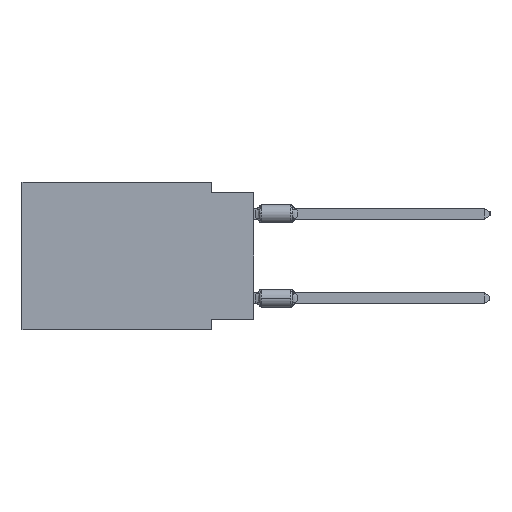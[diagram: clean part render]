
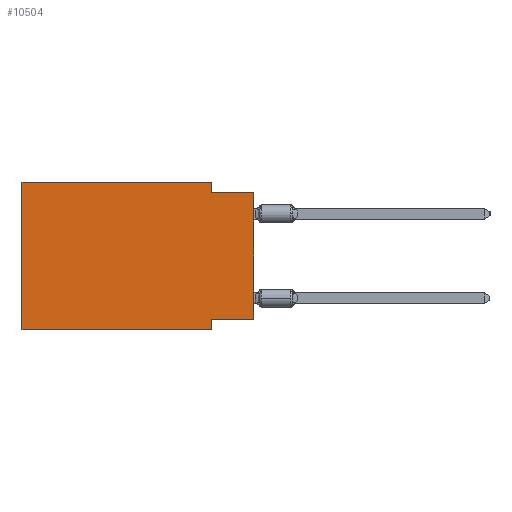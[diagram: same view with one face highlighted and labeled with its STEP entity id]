
A CAD part, left-side view. The second image highlights one B-rep face of the part: STEP entity #10504.
In plain terms, the highlighted planar face has unit normal (-1, 0, 0).
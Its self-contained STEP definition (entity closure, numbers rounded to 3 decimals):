
#73 = VERTEX_POINT ( 'NONE', #5801 ) ;
#1400 = CARTESIAN_POINT ( 'NONE',  ( 0., 13.97, -8.89 ) ) ;
#1407 = CARTESIAN_POINT ( 'NONE',  ( 0., 2.54, 0. ) ) ;
#2314 = EDGE_CURVE ( 'NONE', #11954, #22355, #8105, .T. ) ;
#2711 = ORIENTED_EDGE ( 'NONE', *, *, #22568, .F. ) ;
#4133 = VERTEX_POINT ( 'NONE', #24813 ) ;
#5801 = CARTESIAN_POINT ( 'NONE',  ( 0., 13.97, 0. ) ) ;
#6069 = CARTESIAN_POINT ( 'NONE',  ( 0., 13.97, 0. ) ) ;
#6462 = EDGE_CURVE ( 'NONE', #14252, #42891, #11161, .T. ) ;
#7200 = CARTESIAN_POINT ( 'NONE',  ( 0., 0., 0. ) ) ;
#8105 = LINE ( 'NONE', #1400, #47769 ) ;
#9784 = LINE ( 'NONE', #6069, #10250 ) ;
#9906 = FACE_OUTER_BOUND ( 'NONE', #31492, .T. ) ;
#10010 = EDGE_CURVE ( 'NONE', #11954, #73, #9784, .T. ) ;
#10250 = VECTOR ( 'NONE', #39544, 1000. ) ;
#10504 = ADVANCED_FACE ( 'NONE', ( #9906 ), #32223, .F. ) ;
#11161 = LINE ( 'NONE', #7200, #14114 ) ;
#11415 = ORIENTED_EDGE ( 'NONE', *, *, #10010, .F. ) ;
#11954 = VERTEX_POINT ( 'NONE', #25848 ) ;
#13137 = DIRECTION ( 'NONE',  ( 1., 0., 0. ) ) ;
#13184 = ORIENTED_EDGE ( 'NONE', *, *, #28452, .F. ) ;
#13255 = EDGE_CURVE ( 'NONE', #4133, #22355, #34746, .T. ) ;
#13314 = VERTEX_POINT ( 'NONE', #26338 ) ;
#13627 = CARTESIAN_POINT ( 'NONE',  ( 0., 13.97, 0. ) ) ;
#13911 = LINE ( 'NONE', #17620, #29040 ) ;
#14114 = VECTOR ( 'NONE', #44410, 1000. ) ;
#14252 = VERTEX_POINT ( 'NONE', #45078 ) ;
#14467 = VECTOR ( 'NONE', #22617, 1000. ) ;
#16802 = ORIENTED_EDGE ( 'NONE', *, *, #13255, .F. ) ;
#17620 = CARTESIAN_POINT ( 'NONE',  ( 0., 0., -0.635 ) ) ;
#19489 = DIRECTION ( 'NONE',  ( 0., 0., -1. ) ) ;
#22355 = VERTEX_POINT ( 'NONE', #42960 ) ;
#22568 = EDGE_CURVE ( 'NONE', #14252, #4133, #41195, .T. ) ;
#22617 = DIRECTION ( 'NONE',  ( 0., 0., -1. ) ) ;
#22962 = CARTESIAN_POINT ( 'NONE',  ( 0., 2.54, 0. ) ) ;
#23213 = LINE ( 'NONE', #22962, #37994 ) ;
#24793 = DIRECTION ( 'NONE',  ( 0., 0., -1. ) ) ;
#24813 = CARTESIAN_POINT ( 'NONE',  ( 0., 2.54, -8.255 ) ) ;
#25076 = DIRECTION ( 'NONE',  ( 0., -1., 0. ) ) ;
#25166 = CARTESIAN_POINT ( 'NONE',  ( 0., 0., -0.635 ) ) ;
#25848 = CARTESIAN_POINT ( 'NONE',  ( 0., 13.97, -8.89 ) ) ;
#26311 = CARTESIAN_POINT ( 'NONE',  ( 0., 0., -8.255 ) ) ;
#26338 = CARTESIAN_POINT ( 'NONE',  ( 0., 2.54, -0.635 ) ) ;
#28452 = EDGE_CURVE ( 'NONE', #13314, #42891, #13911, .T. ) ;
#29040 = VECTOR ( 'NONE', #25076, 1000. ) ;
#30043 = CARTESIAN_POINT ( 'NONE',  ( 0., 2.54, -8.89 ) ) ;
#30347 = VERTEX_POINT ( 'NONE', #1407 ) ;
#30642 = CARTESIAN_POINT ( 'NONE',  ( 0., 13.97, 0. ) ) ;
#31492 = EDGE_LOOP ( 'NONE', ( #48617, #13184, #46243, #48714, #11415, #45151, #16802, #2711 ) ) ;
#32223 = PLANE ( 'NONE',  #37193 ) ;
#33463 = VECTOR ( 'NONE', #45398, 1000. ) ;
#34048 = EDGE_CURVE ( 'NONE', #30347, #13314, #23213, .T. ) ;
#34370 = DIRECTION ( 'NONE',  ( 0., -1., 0. ) ) ;
#34397 = VECTOR ( 'NONE', #34370, 1000. ) ;
#34746 = LINE ( 'NONE', #30043, #14467 ) ;
#37193 = AXIS2_PLACEMENT_3D ( 'NONE', #13627, #13137, #24793 ) ;
#37994 = VECTOR ( 'NONE', #19489, 1000. ) ;
#39544 = DIRECTION ( 'NONE',  ( 0., 0., 1. ) ) ;
#41195 = LINE ( 'NONE', #26311, #33463 ) ;
#41837 = DIRECTION ( 'NONE',  ( 0., -1., 0. ) ) ;
#42891 = VERTEX_POINT ( 'NONE', #25166 ) ;
#42960 = CARTESIAN_POINT ( 'NONE',  ( 0., 2.54, -8.89 ) ) ;
#44410 = DIRECTION ( 'NONE',  ( 0., 0., 1. ) ) ;
#45078 = CARTESIAN_POINT ( 'NONE',  ( 0., 0., -8.255 ) ) ;
#45151 = ORIENTED_EDGE ( 'NONE', *, *, #2314, .T. ) ;
#45398 = DIRECTION ( 'NONE',  ( 0., 1., 0. ) ) ;
#45981 = EDGE_CURVE ( 'NONE', #73, #30347, #46275, .T. ) ;
#46243 = ORIENTED_EDGE ( 'NONE', *, *, #34048, .F. ) ;
#46275 = LINE ( 'NONE', #30642, #34397 ) ;
#47769 = VECTOR ( 'NONE', #41837, 1000. ) ;
#48617 = ORIENTED_EDGE ( 'NONE', *, *, #6462, .T. ) ;
#48714 = ORIENTED_EDGE ( 'NONE', *, *, #45981, .F. ) ;
